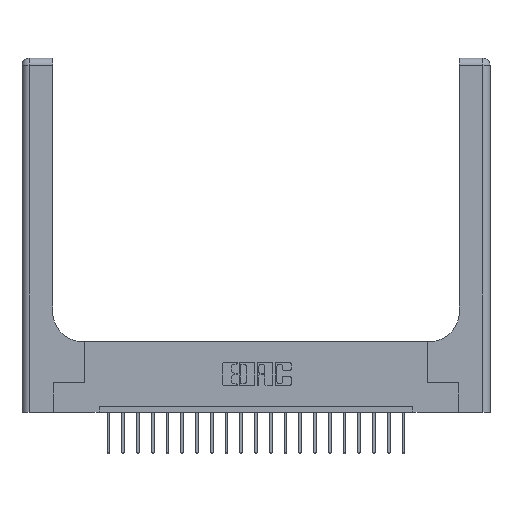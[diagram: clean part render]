
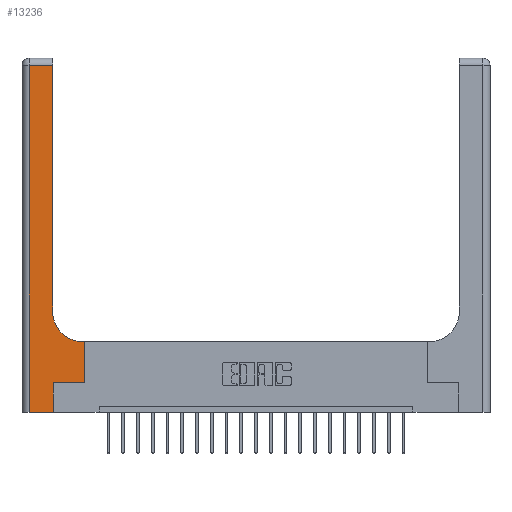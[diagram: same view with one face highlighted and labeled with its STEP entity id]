
A CAD part, top view. The second image highlights one B-rep face of the part: STEP entity #13236.
In plain terms, the highlighted planar face has unit normal (0, 0, 1).
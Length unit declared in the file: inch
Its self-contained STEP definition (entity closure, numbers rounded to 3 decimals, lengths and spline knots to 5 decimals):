
#45 = VERTEX_POINT ( 'NONE', #4421 ) ;
#152 = DIRECTION ( 'NONE',  ( -1., 0., 0. ) ) ;
#922 = CARTESIAN_POINT ( 'NONE',  ( 0.51, 0.85, 0.37 ) ) ;
#941 = ORIENTED_EDGE ( 'NONE', *, *, #19630, .T. ) ;
#1223 = VERTEX_POINT ( 'NONE', #5865 ) ;
#1405 = ORIENTED_EDGE ( 'NONE', *, *, #12364, .T. ) ;
#1615 = VERTEX_POINT ( 'NONE', #3719 ) ;
#1676 = DIRECTION ( 'NONE',  ( 0., 0., -1. ) ) ;
#1762 = VECTOR ( 'NONE', #11882, 39.37008 ) ;
#2324 = ORIENTED_EDGE ( 'NONE', *, *, #5303, .T. ) ;
#2632 = ORIENTED_EDGE ( 'NONE', *, *, #4384, .T. ) ;
#2666 = VERTEX_POINT ( 'NONE', #6400 ) ;
#2866 = LINE ( 'NONE', #14931, #8997 ) ;
#3100 = EDGE_CURVE ( 'NONE', #15367, #6687, #15697, .T. ) ;
#3429 = EDGE_LOOP ( 'NONE', ( #1405, #12037, #941, #6358, #19895, #10723, #2632, #14548, #2324 ) ) ;
#3719 = CARTESIAN_POINT ( 'NONE',  ( 0.26, 2.94, 0.37 ) ) ;
#4067 = VECTOR ( 'NONE', #9944, 39.37008 ) ;
#4240 = VECTOR ( 'NONE', #15868, 39.37008 ) ;
#4291 = CARTESIAN_POINT ( 'NONE',  ( 0.528, 0.25, 0.37 ) ) ;
#4384 = EDGE_CURVE ( 'NONE', #11719, #1223, #18699, .T. ) ;
#4421 = CARTESIAN_POINT ( 'NONE',  ( 0.06, 2.94, 0.37 ) ) ;
#5303 = EDGE_CURVE ( 'NONE', #13872, #2666, #5763, .T. ) ;
#5763 = CIRCLE ( 'NONE', #16500, 0.25 ) ;
#5865 = CARTESIAN_POINT ( 'NONE',  ( 0.528, 0.6, 0.37 ) ) ;
#6358 = ORIENTED_EDGE ( 'NONE', *, *, #3100, .T. ) ;
#6400 = CARTESIAN_POINT ( 'NONE',  ( 0.26, 0.85, 0.37 ) ) ;
#6536 = CARTESIAN_POINT ( 'NONE',  ( 0.528, 0.25, 0.37 ) ) ;
#6687 = VERTEX_POINT ( 'NONE', #17272 ) ;
#7587 = EDGE_CURVE ( 'NONE', #16859, #11719, #10080, .T. ) ;
#7588 = LINE ( 'NONE', #18595, #14157 ) ;
#7999 = DIRECTION ( 'NONE',  ( 0., 1., 0. ) ) ;
#8980 = LINE ( 'NONE', #9561, #12263 ) ;
#8997 = VECTOR ( 'NONE', #11906, 39.37008 ) ;
#9188 = DIRECTION ( 'NONE',  ( 1., 0., 0. ) ) ;
#9561 = CARTESIAN_POINT ( 'NONE',  ( 0.265, 0., 0.37 ) ) ;
#9914 = PLANE ( 'NONE',  #19471 ) ;
#9944 = DIRECTION ( 'NONE',  ( 1., 0., 0. ) ) ;
#10080 = LINE ( 'NONE', #11006, #4240 ) ;
#10166 = EDGE_CURVE ( 'NONE', #6687, #16859, #8980, .T. ) ;
#10723 = ORIENTED_EDGE ( 'NONE', *, *, #7587, .T. ) ;
#10925 = DIRECTION ( 'NONE',  ( 0., 1., 0. ) ) ;
#11006 = CARTESIAN_POINT ( 'NONE',  ( 0.265, 0.25, 0.37 ) ) ;
#11235 = DIRECTION ( 'NONE',  ( 0., 1., 0. ) ) ;
#11400 = CARTESIAN_POINT ( 'NONE',  ( 0., 3., 0.37 ) ) ;
#11543 = CARTESIAN_POINT ( 'NONE',  ( 0.06, 0., 0.37 ) ) ;
#11719 = VERTEX_POINT ( 'NONE', #4291 ) ;
#11882 = DIRECTION ( 'NONE',  ( 0., -1., 0. ) ) ;
#11906 = DIRECTION ( 'NONE',  ( -1., 0., 0. ) ) ;
#12037 = ORIENTED_EDGE ( 'NONE', *, *, #19632, .T. ) ;
#12096 = CARTESIAN_POINT ( 'NONE',  ( 0.06, 3., 0.37 ) ) ;
#12263 = VECTOR ( 'NONE', #7999, 39.37008 ) ;
#12272 = CARTESIAN_POINT ( 'NONE',  ( 0., 0., 0.37 ) ) ;
#12364 = EDGE_CURVE ( 'NONE', #2666, #1615, #20571, .T. ) ;
#12761 = EDGE_CURVE ( 'NONE', #1223, #13872, #2866, .T. ) ;
#13236 = ADVANCED_FACE ( 'NONE', ( #19979 ), #9914, .F. ) ;
#13622 = DIRECTION ( 'NONE',  ( -1., 0., 0. ) ) ;
#13872 = VERTEX_POINT ( 'NONE', #20230 ) ;
#14105 = CARTESIAN_POINT ( 'NONE',  ( 0.26, 3., 0.37 ) ) ;
#14157 = VECTOR ( 'NONE', #13622, 39.37008 ) ;
#14548 = ORIENTED_EDGE ( 'NONE', *, *, #12761, .T. ) ;
#14931 = CARTESIAN_POINT ( 'NONE',  ( 0.26, 0.6, 0.37 ) ) ;
#15367 = VERTEX_POINT ( 'NONE', #11543 ) ;
#15697 = LINE ( 'NONE', #12272, #4067 ) ;
#15868 = DIRECTION ( 'NONE',  ( 1., 0., 0. ) ) ;
#15968 = VECTOR ( 'NONE', #10925, 39.37008 ) ;
#16500 = AXIS2_PLACEMENT_3D ( 'NONE', #922, #20308, #9188 ) ;
#16859 = VERTEX_POINT ( 'NONE', #17284 ) ;
#17272 = CARTESIAN_POINT ( 'NONE',  ( 0.265, 0., 0.37 ) ) ;
#17284 = CARTESIAN_POINT ( 'NONE',  ( 0.265, 0.25, 0.37 ) ) ;
#17908 = LINE ( 'NONE', #12096, #1762 ) ;
#18595 = CARTESIAN_POINT ( 'NONE',  ( 0., 2.94, 0.37 ) ) ;
#18699 = LINE ( 'NONE', #6536, #18951 ) ;
#18951 = VECTOR ( 'NONE', #11235, 39.37008 ) ;
#19471 = AXIS2_PLACEMENT_3D ( 'NONE', #11400, #1676, #152 ) ;
#19630 = EDGE_CURVE ( 'NONE', #45, #15367, #17908, .T. ) ;
#19632 = EDGE_CURVE ( 'NONE', #1615, #45, #7588, .T. ) ;
#19895 = ORIENTED_EDGE ( 'NONE', *, *, #10166, .T. ) ;
#19979 = FACE_OUTER_BOUND ( 'NONE', #3429, .T. ) ;
#20230 = CARTESIAN_POINT ( 'NONE',  ( 0.51, 0.6, 0.37 ) ) ;
#20308 = DIRECTION ( 'NONE',  ( 0., 0., -1. ) ) ;
#20571 = LINE ( 'NONE', #14105, #15968 ) ;
